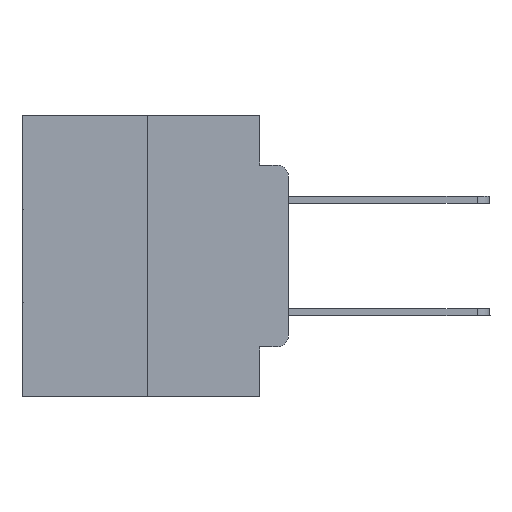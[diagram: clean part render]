
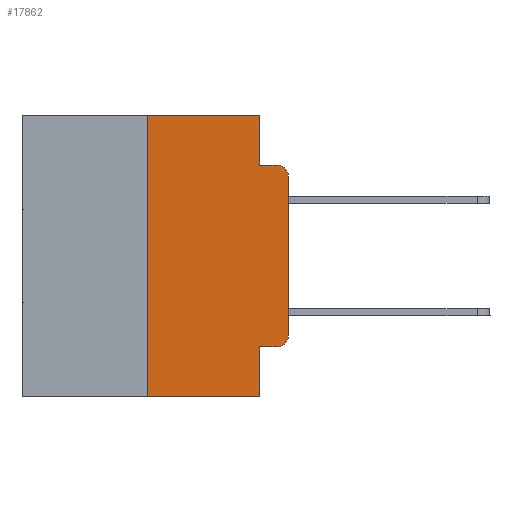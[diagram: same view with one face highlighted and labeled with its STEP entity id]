
A CAD part, left-side view. The second image highlights one B-rep face of the part: STEP entity #17862.
In plain terms, the highlighted planar face has unit normal (-1, 0, 0).
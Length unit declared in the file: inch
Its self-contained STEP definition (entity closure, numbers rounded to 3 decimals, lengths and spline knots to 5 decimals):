
#110 = LINE ( 'NONE', #14032, #3381 ) ;
#1070 = CARTESIAN_POINT ( 'NONE',  ( 0., 0.051, 0. ) ) ;
#1684 = VECTOR ( 'NONE', #23935, 39.37008 ) ;
#2109 = CARTESIAN_POINT ( 'NONE',  ( 0., 0.25, 0. ) ) ;
#2737 = VERTEX_POINT ( 'NONE', #21510 ) ;
#3131 = LINE ( 'NONE', #10138, #1684 ) ;
#3381 = VECTOR ( 'NONE', #4729, 39.37008 ) ;
#3402 = VERTEX_POINT ( 'NONE', #5378 ) ;
#3498 = ORIENTED_EDGE ( 'NONE', *, *, #24914, .T. ) ;
#3969 = CARTESIAN_POINT ( 'NONE',  ( 0., 0., 0. ) ) ;
#4452 = CARTESIAN_POINT ( 'NONE',  ( 0., 0.473, 0. ) ) ;
#4641 = CARTESIAN_POINT ( 'NONE',  ( 0., 0.051, -0.5 ) ) ;
#4729 = DIRECTION ( 'NONE',  ( 0., -1., 0. ) ) ;
#5359 = CARTESIAN_POINT ( 'NONE',  ( 0., 0.02, -0.1085 ) ) ;
#5378 = CARTESIAN_POINT ( 'NONE',  ( 0., 0.25, 0. ) ) ;
#5834 = CARTESIAN_POINT ( 'NONE',  ( 0., 0.051, 0. ) ) ;
#6704 = EDGE_CURVE ( 'NONE', #24535, #7247, #7798, .T. ) ;
#7247 = VERTEX_POINT ( 'NONE', #20073 ) ;
#7505 = AXIS2_PLACEMENT_3D ( 'NONE', #26051, #9635, #28491 ) ;
#7685 = EDGE_CURVE ( 'NONE', #2737, #19743, #22229, .T. ) ;
#7798 = LINE ( 'NONE', #5834, #19020 ) ;
#9635 = DIRECTION ( 'NONE',  ( 1., 0., 0. ) ) ;
#10138 = CARTESIAN_POINT ( 'NONE',  ( 0., 0.051, -0.0885 ) ) ;
#10272 = LINE ( 'NONE', #19598, #19329 ) ;
#10668 = EDGE_CURVE ( 'NONE', #23177, #15503, #18041, .T. ) ;
#10765 = ORIENTED_EDGE ( 'NONE', *, *, #27039, .T. ) ;
#10993 = CARTESIAN_POINT ( 'NONE',  ( 0., 0.25, -0.5 ) ) ;
#11075 = ORIENTED_EDGE ( 'NONE', *, *, #25171, .F. ) ;
#11369 = DIRECTION ( 'NONE',  ( 0., -1., 0. ) ) ;
#11517 = DIRECTION ( 'NONE',  ( 0., 0., -1. ) ) ;
#11810 = VERTEX_POINT ( 'NONE', #10993 ) ;
#12718 = LINE ( 'NONE', #2109, #21426 ) ;
#12949 = LINE ( 'NONE', #3969, #30026 ) ;
#13527 = ORIENTED_EDGE ( 'NONE', *, *, #14625, .F. ) ;
#14032 = CARTESIAN_POINT ( 'NONE',  ( 0., 0.473, -0.5 ) ) ;
#14260 = EDGE_CURVE ( 'NONE', #11810, #3402, #12718, .T. ) ;
#14282 = VERTEX_POINT ( 'NONE', #4641 ) ;
#14625 = EDGE_CURVE ( 'NONE', #23385, #14282, #21067, .T. ) ;
#14942 = ORIENTED_EDGE ( 'NONE', *, *, #6704, .F. ) ;
#15151 = EDGE_LOOP ( 'NONE', ( #3498, #26657, #11075, #14942, #18901, #16923, #22492, #13527, #10765, #17938 ) ) ;
#15308 = DIRECTION ( 'NONE',  ( 0., -1., 0. ) ) ;
#15503 = VERTEX_POINT ( 'NONE', #22328 ) ;
#16231 = CARTESIAN_POINT ( 'NONE',  ( 0., 0.02, -0.0885 ) ) ;
#16246 = CARTESIAN_POINT ( 'NONE',  ( 0., 0.02, -0.3915 ) ) ;
#16335 = CARTESIAN_POINT ( 'NONE',  ( 0., 0.051, 0. ) ) ;
#16705 = DIRECTION ( 'NONE',  ( -1., 0., 0. ) ) ;
#16800 = DIRECTION ( 'NONE',  ( 0., 0., -1. ) ) ;
#16923 = ORIENTED_EDGE ( 'NONE', *, *, #14260, .F. ) ;
#17283 = DIRECTION ( 'NONE',  ( 0., 0., -1. ) ) ;
#17862 = ADVANCED_FACE ( 'NONE', ( #19089 ), #23722, .F. ) ;
#17938 = ORIENTED_EDGE ( 'NONE', *, *, #10668, .T. ) ;
#18041 = CIRCLE ( 'NONE', #22878, 0.02 ) ;
#18901 = ORIENTED_EDGE ( 'NONE', *, *, #29300, .F. ) ;
#19020 = VECTOR ( 'NONE', #26827, 39.37008 ) ;
#19089 = FACE_OUTER_BOUND ( 'NONE', #15151, .T. ) ;
#19154 = CARTESIAN_POINT ( 'NONE',  ( 0., 0.051, -0.4115 ) ) ;
#19329 = VECTOR ( 'NONE', #15308, 39.37008 ) ;
#19598 = CARTESIAN_POINT ( 'NONE',  ( 0., 0.051, -0.4115 ) ) ;
#19743 = VERTEX_POINT ( 'NONE', #16231 ) ;
#20073 = CARTESIAN_POINT ( 'NONE',  ( 0., 0.051, -0.0885 ) ) ;
#20375 = VECTOR ( 'NONE', #11369, 39.37008 ) ;
#21067 = LINE ( 'NONE', #1070, #23589 ) ;
#21426 = VECTOR ( 'NONE', #27667, 39.37008 ) ;
#21510 = CARTESIAN_POINT ( 'NONE',  ( 0., 0., -0.1085 ) ) ;
#22229 = CIRCLE ( 'NONE', #23002, 0.02 ) ;
#22328 = CARTESIAN_POINT ( 'NONE',  ( 0., 0., -0.3915 ) ) ;
#22492 = ORIENTED_EDGE ( 'NONE', *, *, #27948, .T. ) ;
#22837 = CARTESIAN_POINT ( 'NONE',  ( 0., 0.02, -0.4115 ) ) ;
#22878 = AXIS2_PLACEMENT_3D ( 'NONE', #16246, #23061, #11517 ) ;
#23002 = AXIS2_PLACEMENT_3D ( 'NONE', #5359, #16705, #16800 ) ;
#23061 = DIRECTION ( 'NONE',  ( -1., 0., 0. ) ) ;
#23177 = VERTEX_POINT ( 'NONE', #22837 ) ;
#23385 = VERTEX_POINT ( 'NONE', #19154 ) ;
#23589 = VECTOR ( 'NONE', #17283, 39.37008 ) ;
#23722 = PLANE ( 'NONE',  #7505 ) ;
#23935 = DIRECTION ( 'NONE',  ( 0., -1., 0. ) ) ;
#24535 = VERTEX_POINT ( 'NONE', #16335 ) ;
#24914 = EDGE_CURVE ( 'NONE', #15503, #2737, #12949, .T. ) ;
#25171 = EDGE_CURVE ( 'NONE', #7247, #19743, #3131, .T. ) ;
#26051 = CARTESIAN_POINT ( 'NONE',  ( 0., 0.473, 0. ) ) ;
#26657 = ORIENTED_EDGE ( 'NONE', *, *, #7685, .T. ) ;
#26827 = DIRECTION ( 'NONE',  ( 0., 0., -1. ) ) ;
#27039 = EDGE_CURVE ( 'NONE', #23385, #23177, #10272, .T. ) ;
#27667 = DIRECTION ( 'NONE',  ( 0., 0., 1. ) ) ;
#27948 = EDGE_CURVE ( 'NONE', #11810, #14282, #110, .T. ) ;
#27993 = LINE ( 'NONE', #4452, #20375 ) ;
#28491 = DIRECTION ( 'NONE',  ( 0., 0., -1. ) ) ;
#29300 = EDGE_CURVE ( 'NONE', #3402, #24535, #27993, .T. ) ;
#29342 = DIRECTION ( 'NONE',  ( 0., 0., 1. ) ) ;
#30026 = VECTOR ( 'NONE', #29342, 39.37008 ) ;
